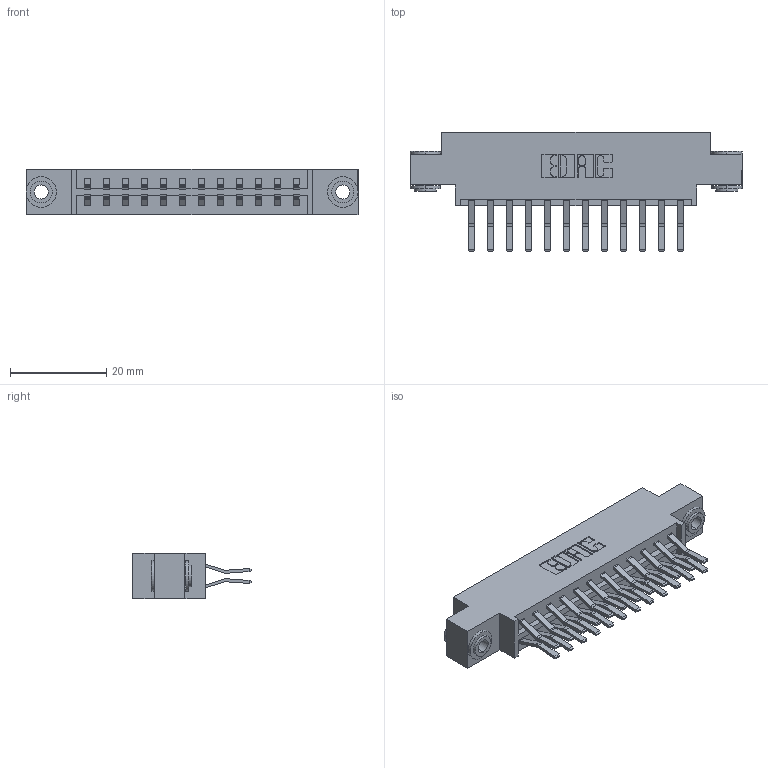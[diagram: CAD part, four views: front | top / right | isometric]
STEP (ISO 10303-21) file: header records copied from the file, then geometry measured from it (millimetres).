
FILE_DESCRIPTION (( 'STEP AP203' ), '1' );
FILE_NAME ('833-024-560-803.STEP', '2020-06-01T22:54:26', ( '' ), ( '' ), 'SwSTEP 2.0', 'SolidWorks 2020', '' );
FILE_SCHEMA (( 'CONFIG_CONTROL_DESIGN' ));
Length unit declared in the file: inch
Products named in the file (4): 833 Part_Offset - .156 Dia - TH; 345-250-002_345-250-002-102; 833-024-560-803; 345-292-001_560 Tail
Assembly tree (27 placements, depth 2):
  833-024-560-803
    833 Part_Offset - .156 Dia - TH
    345-292-001_560 Tail  x24
    345-250-002_345-250-002-102  x2
Bounding box: 69.09 x 24.78 x 9.4 mm (x, y, z)
Volume: 6721.8 mm3; surface area: 8515 mm2
Topology: 27 solids, 27 shells, 1452 faces, 4263 edges, 2806 vertices
Faces by surface type: plane 948, cylinder 496, cone 8
Entity records: 12470 total; most frequent: CARTESIAN_POINT 2081, ORIENTED_EDGE 2010, DIRECTION 1867, EDGE_CURVE 1005, LINE 849, VECTOR 849, VERTEX_POINT 666, AXIS2_PLACEMENT_3D 509
